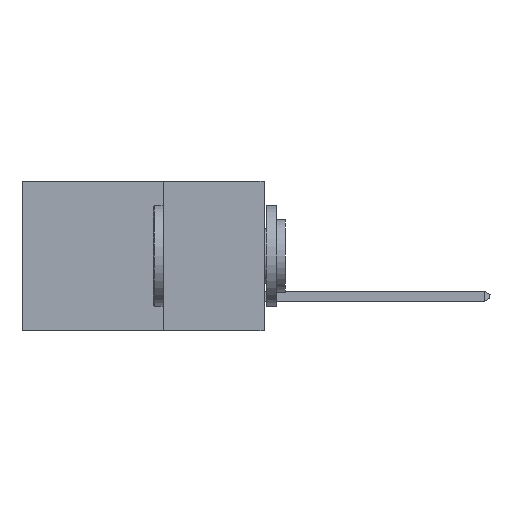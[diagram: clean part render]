
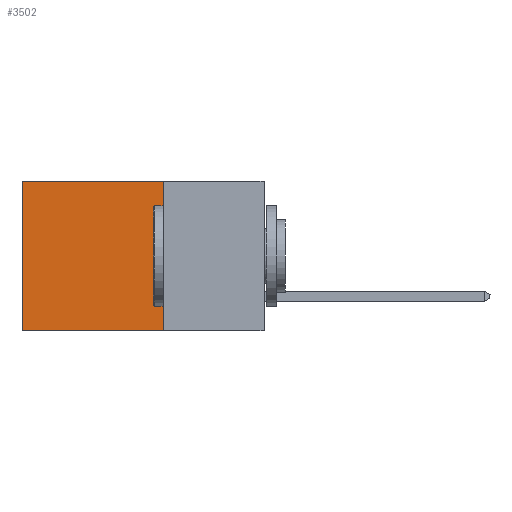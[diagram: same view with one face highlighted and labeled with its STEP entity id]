
A CAD part, left-side view. The second image highlights one B-rep face of the part: STEP entity #3502.
In plain terms, the highlighted planar face has unit normal (-1, 0, 0).
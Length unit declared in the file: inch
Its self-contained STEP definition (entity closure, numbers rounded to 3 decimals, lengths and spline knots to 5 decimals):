
#267 = CARTESIAN_POINT ( 'NONE',  ( 0.298, 0.25, 0. ) ) ;
#331 = DIRECTION ( 'NONE',  ( 1., 0., 0. ) ) ;
#904 = VECTOR ( 'NONE', #12310, 39.37008 ) ;
#982 = ORIENTED_EDGE ( 'NONE', *, *, #14993, .T. ) ;
#2529 = CARTESIAN_POINT ( 'NONE',  ( 0.298, 0.25, 0. ) ) ;
#2651 = VERTEX_POINT ( 'NONE', #4139 ) ;
#2814 = VECTOR ( 'NONE', #13299, 39.37008 ) ;
#3402 = CARTESIAN_POINT ( 'NONE',  ( 0.298, 0.6, 0. ) ) ;
#3502 = ADVANCED_FACE ( 'NONE', ( #13361 ), #5015, .F. ) ;
#3652 = DIRECTION ( 'NONE',  ( 0., 0., -1. ) ) ;
#4139 = CARTESIAN_POINT ( 'NONE',  ( 0.298, 0.6, 0. ) ) ;
#5015 = PLANE ( 'NONE',  #16381 ) ;
#5109 = CARTESIAN_POINT ( 'NONE',  ( 0.298, 0.6, -0.37 ) ) ;
#5471 = LINE ( 'NONE', #3402, #2814 ) ;
#5596 = VERTEX_POINT ( 'NONE', #18002 ) ;
#6615 = CARTESIAN_POINT ( 'NONE',  ( 0.298, 0.25, 0. ) ) ;
#7858 = ORIENTED_EDGE ( 'NONE', *, *, #16354, .T. ) ;
#8954 = EDGE_CURVE ( 'NONE', #16396, #5596, #18234, .T. ) ;
#9831 = VERTEX_POINT ( 'NONE', #5109 ) ;
#10257 = VECTOR ( 'NONE', #15446, 39.37008 ) ;
#11227 = ORIENTED_EDGE ( 'NONE', *, *, #11240, .F. ) ;
#11240 = EDGE_CURVE ( 'NONE', #5596, #9831, #12476, .T. ) ;
#12310 = DIRECTION ( 'NONE',  ( 0., 0., -1. ) ) ;
#12476 = LINE ( 'NONE', #14144, #10257 ) ;
#13299 = DIRECTION ( 'NONE',  ( 0., 0., -1. ) ) ;
#13361 = FACE_OUTER_BOUND ( 'NONE', #18309, .T. ) ;
#13683 = DIRECTION ( 'NONE',  ( 0., 1., 0. ) ) ;
#14144 = CARTESIAN_POINT ( 'NONE',  ( 0.298, 0.25, -0.37 ) ) ;
#14993 = EDGE_CURVE ( 'NONE', #2651, #9831, #5471, .T. ) ;
#15310 = LINE ( 'NONE', #16632, #15619 ) ;
#15446 = DIRECTION ( 'NONE',  ( 0., 1., 0. ) ) ;
#15619 = VECTOR ( 'NONE', #13683, 39.37008 ) ;
#16354 = EDGE_CURVE ( 'NONE', #16396, #2651, #15310, .T. ) ;
#16381 = AXIS2_PLACEMENT_3D ( 'NONE', #267, #331, #3652 ) ;
#16396 = VERTEX_POINT ( 'NONE', #2529 ) ;
#16632 = CARTESIAN_POINT ( 'NONE',  ( 0.298, 0.25, 0. ) ) ;
#17007 = ORIENTED_EDGE ( 'NONE', *, *, #8954, .F. ) ;
#18002 = CARTESIAN_POINT ( 'NONE',  ( 0.298, 0.25, -0.37 ) ) ;
#18234 = LINE ( 'NONE', #6615, #904 ) ;
#18309 = EDGE_LOOP ( 'NONE', ( #982, #11227, #17007, #7858 ) ) ;
